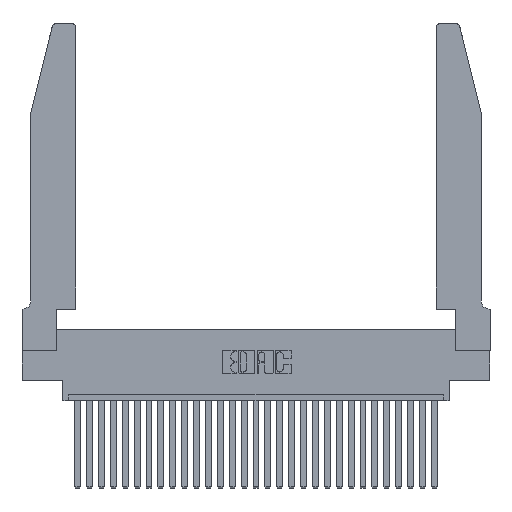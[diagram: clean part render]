
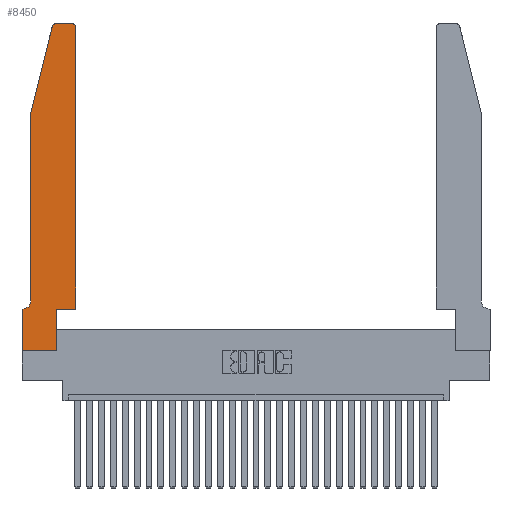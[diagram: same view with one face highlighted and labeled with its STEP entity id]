
A CAD part, top view. The second image highlights one B-rep face of the part: STEP entity #8450.
In plain terms, the highlighted planar face has unit normal (0, 0, 1).
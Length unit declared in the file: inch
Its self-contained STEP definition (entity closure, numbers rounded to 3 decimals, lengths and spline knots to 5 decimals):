
#739 = CARTESIAN_POINT ( 'NONE',  ( 0.0055, 0.42, 0.37 ) ) ;
#827 = DIRECTION ( 'NONE',  ( 0., 1., 0. ) ) ;
#961 = CARTESIAN_POINT ( 'NONE',  ( 0., 0., 0.37 ) ) ;
#1421 = DIRECTION ( 'NONE',  ( 1., 0., 0. ) ) ;
#1999 = LINE ( 'NONE', #16637, #16292 ) ;
#2106 = VERTEX_POINT ( 'NONE', #14287 ) ;
#2362 = EDGE_CURVE ( 'NONE', #26756, #17062, #14995, .T. ) ;
#3024 = DIRECTION ( 'NONE',  ( 0., 0., -1. ) ) ;
#3545 = VECTOR ( 'NONE', #16910, 39.37008 ) ;
#3790 = DIRECTION ( 'NONE',  ( 1., 0., 0. ) ) ;
#3862 = VERTEX_POINT ( 'NONE', #25218 ) ;
#4416 = VECTOR ( 'NONE', #19972, 39.37008 ) ;
#4655 = EDGE_CURVE ( 'NONE', #23447, #17879, #1999, .T. ) ;
#5315 = CARTESIAN_POINT ( 'NONE',  ( 0.0755, 2., 0.37 ) ) ;
#5375 = EDGE_CURVE ( 'NONE', #29190, #26756, #10489, .T. ) ;
#6209 = DIRECTION ( 'NONE',  ( 0., 1., 0. ) ) ;
#6262 = CARTESIAN_POINT ( 'NONE',  ( 0.0055, 0.35, 0.37 ) ) ;
#6502 = CARTESIAN_POINT ( 'NONE',  ( 0., 0., 0.37 ) ) ;
#6647 = CARTESIAN_POINT ( 'NONE',  ( 0.4205, 2.75, 0.37 ) ) ;
#7106 = CARTESIAN_POINT ( 'NONE',  ( 0., 0.35, 0.37 ) ) ;
#7128 = EDGE_CURVE ( 'NONE', #2106, #29190, #10058, .T. ) ;
#7803 = CARTESIAN_POINT ( 'NONE',  ( 0.2865, 0.35, 0.37 ) ) ;
#8450 = ADVANCED_FACE ( 'NONE', ( #12875 ), #20397, .T. ) ;
#8757 = ORIENTED_EDGE ( 'NONE', *, *, #28504, .T. ) ;
#8779 = ORIENTED_EDGE ( 'NONE', *, *, #20371, .T. ) ;
#8806 = DIRECTION ( 'NONE',  ( 0., -1., 0. ) ) ;
#9452 = ORIENTED_EDGE ( 'NONE', *, *, #19871, .T. ) ;
#10058 = CIRCLE ( 'NONE', #19267, 0.03 ) ;
#10060 = CARTESIAN_POINT ( 'NONE',  ( 0.2865, 0., 0.37 ) ) ;
#10461 = EDGE_CURVE ( 'NONE', #17879, #2106, #19551, .T. ) ;
#10464 = DIRECTION ( 'NONE',  ( -1., 0., 0. ) ) ;
#10489 = LINE ( 'NONE', #19873, #4416 ) ;
#10610 = LINE ( 'NONE', #6502, #22416 ) ;
#11038 = LINE ( 'NONE', #961, #3545 ) ;
#11096 = ORIENTED_EDGE ( 'NONE', *, *, #4655, .T. ) ;
#11100 = VERTEX_POINT ( 'NONE', #29376 ) ;
#11245 = LINE ( 'NONE', #7803, #28688 ) ;
#11414 = DIRECTION ( 'NONE',  ( 1., 0., 0. ) ) ;
#11609 = ORIENTED_EDGE ( 'NONE', *, *, #5375, .T. ) ;
#11942 = ORIENTED_EDGE ( 'NONE', *, *, #2362, .T. ) ;
#12875 = FACE_OUTER_BOUND ( 'NONE', #16697, .T. ) ;
#12880 = CARTESIAN_POINT ( 'NONE',  ( 0., 0.35, 0.37 ) ) ;
#13224 = CARTESIAN_POINT ( 'NONE',  ( 0.4505, 0.35, 0.37 ) ) ;
#13381 = VERTEX_POINT ( 'NONE', #10060 ) ;
#13625 = VERTEX_POINT ( 'NONE', #6262 ) ;
#13650 = VERTEX_POINT ( 'NONE', #12880 ) ;
#13738 = ORIENTED_EDGE ( 'NONE', *, *, #27391, .T. ) ;
#14177 = AXIS2_PLACEMENT_3D ( 'NONE', #7106, #18195, #11414 ) ;
#14287 = CARTESIAN_POINT ( 'NONE',  ( 0.4505, 2.72, 0.37 ) ) ;
#14698 = AXIS2_PLACEMENT_3D ( 'NONE', #17451, #15353, #17743 ) ;
#14995 = CIRCLE ( 'NONE', #14698, 0.03 ) ;
#15016 = CARTESIAN_POINT ( 'NONE',  ( 0.2865, 0.35, 0.37 ) ) ;
#15353 = DIRECTION ( 'NONE',  ( 0., 0., 1. ) ) ;
#16292 = VECTOR ( 'NONE', #17121, 39.37008 ) ;
#16347 = VECTOR ( 'NONE', #10464, 39.37008 ) ;
#16564 = VECTOR ( 'NONE', #8806, 39.37008 ) ;
#16637 = CARTESIAN_POINT ( 'NONE',  ( 0.4505, 0.35, 0.37 ) ) ;
#16697 = EDGE_LOOP ( 'NONE', ( #11609, #11942, #25336, #17365, #9452, #13738, #8779, #28586, #8757, #11096, #25063, #23062 ) ) ;
#16910 = DIRECTION ( 'NONE',  ( 0., -1., 0. ) ) ;
#17062 = VERTEX_POINT ( 'NONE', #24470 ) ;
#17087 = EDGE_CURVE ( 'NONE', #3862, #11100, #19425, .T. ) ;
#17121 = DIRECTION ( 'NONE',  ( 1., 0., 0. ) ) ;
#17365 = ORIENTED_EDGE ( 'NONE', *, *, #17087, .T. ) ;
#17403 = VERTEX_POINT ( 'NONE', #21226 ) ;
#17451 = CARTESIAN_POINT ( 'NONE',  ( 0.284, 2.72, 0.37 ) ) ;
#17478 = CARTESIAN_POINT ( 'NONE',  ( 0.4205, 2.72, 0.37 ) ) ;
#17743 = DIRECTION ( 'NONE',  ( 1., 0., 0. ) ) ;
#17860 = CIRCLE ( 'NONE', #27491, 0.07 ) ;
#17879 = VERTEX_POINT ( 'NONE', #21192 ) ;
#18195 = DIRECTION ( 'NONE',  ( 0., 0., 1. ) ) ;
#18985 = DIRECTION ( 'NONE',  ( -1., 0., 0. ) ) ;
#19267 = AXIS2_PLACEMENT_3D ( 'NONE', #17478, #22245, #3790 ) ;
#19425 = LINE ( 'NONE', #22490, #16564 ) ;
#19551 = LINE ( 'NONE', #13224, #25601 ) ;
#19871 = EDGE_CURVE ( 'NONE', #11100, #13625, #17860, .T. ) ;
#19873 = CARTESIAN_POINT ( 'NONE',  ( 0.2605, 2.75, 0.37 ) ) ;
#19972 = DIRECTION ( 'NONE',  ( -1., 0., 0. ) ) ;
#20371 = EDGE_CURVE ( 'NONE', #13650, #17403, #11038, .T. ) ;
#20397 = PLANE ( 'NONE',  #14177 ) ;
#21192 = CARTESIAN_POINT ( 'NONE',  ( 0.4505, 0.35, 0.37 ) ) ;
#21219 = EDGE_CURVE ( 'NONE', #17403, #13381, #10610, .T. ) ;
#21226 = CARTESIAN_POINT ( 'NONE',  ( 0., 0., 0.37 ) ) ;
#22245 = DIRECTION ( 'NONE',  ( 0., 0., 1. ) ) ;
#22411 = LINE ( 'NONE', #26713, #16347 ) ;
#22416 = VECTOR ( 'NONE', #1421, 39.37008 ) ;
#22490 = CARTESIAN_POINT ( 'NONE',  ( 0.0755, 2., 0.37 ) ) ;
#22703 = LINE ( 'NONE', #5315, #24116 ) ;
#23062 = ORIENTED_EDGE ( 'NONE', *, *, #7128, .T. ) ;
#23447 = VERTEX_POINT ( 'NONE', #15016 ) ;
#24116 = VECTOR ( 'NONE', #25848, 39.37008 ) ;
#24470 = CARTESIAN_POINT ( 'NONE',  ( 0.25487, 2.72718, 0.37 ) ) ;
#25063 = ORIENTED_EDGE ( 'NONE', *, *, #10461, .T. ) ;
#25218 = CARTESIAN_POINT ( 'NONE',  ( 0.0755, 2., 0.37 ) ) ;
#25336 = ORIENTED_EDGE ( 'NONE', *, *, #28436, .T. ) ;
#25601 = VECTOR ( 'NONE', #6209, 39.37008 ) ;
#25848 = DIRECTION ( 'NONE',  ( -0.239, -0.971, 0. ) ) ;
#26261 = CARTESIAN_POINT ( 'NONE',  ( 0.284, 2.75, 0.37 ) ) ;
#26713 = CARTESIAN_POINT ( 'NONE',  ( 0.0755, 0.35, 0.37 ) ) ;
#26756 = VERTEX_POINT ( 'NONE', #26261 ) ;
#27391 = EDGE_CURVE ( 'NONE', #13625, #13650, #22411, .T. ) ;
#27491 = AXIS2_PLACEMENT_3D ( 'NONE', #739, #3024, #18985 ) ;
#28436 = EDGE_CURVE ( 'NONE', #17062, #3862, #22703, .T. ) ;
#28504 = EDGE_CURVE ( 'NONE', #13381, #23447, #11245, .T. ) ;
#28586 = ORIENTED_EDGE ( 'NONE', *, *, #21219, .T. ) ;
#28688 = VECTOR ( 'NONE', #827, 39.37008 ) ;
#29190 = VERTEX_POINT ( 'NONE', #6647 ) ;
#29376 = CARTESIAN_POINT ( 'NONE',  ( 0.0755, 0.42, 0.37 ) ) ;
